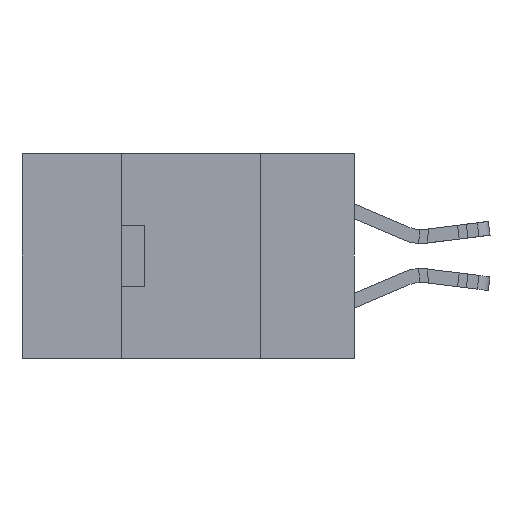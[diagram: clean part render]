
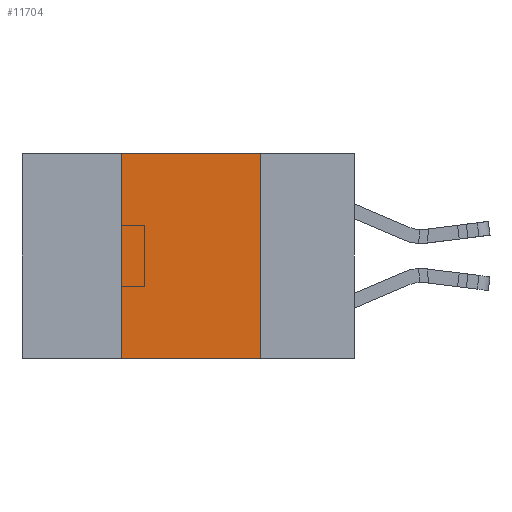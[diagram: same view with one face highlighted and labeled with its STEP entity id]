
A CAD part, left-side view. The second image highlights one B-rep face of the part: STEP entity #11704.
In plain terms, the highlighted planar face has unit normal (-1, 0, 0).
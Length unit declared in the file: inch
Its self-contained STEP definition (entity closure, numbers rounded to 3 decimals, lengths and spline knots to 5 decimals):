
#1423 = DIRECTION ( 'NONE',  ( 0., 0., -1. ) ) ;
#1690 = CARTESIAN_POINT ( 'NONE',  ( 0., 0.42, -0.37 ) ) ;
#1704 = DIRECTION ( 'NONE',  ( 1., 0., 0. ) ) ;
#2603 = EDGE_CURVE ( 'NONE', #26411, #3681, #3736, .T. ) ;
#2854 = VECTOR ( 'NONE', #8076, 39.37008 ) ;
#3369 = ORIENTED_EDGE ( 'NONE', *, *, #2603, .F. ) ;
#3681 = VERTEX_POINT ( 'NONE', #10088 ) ;
#3736 = LINE ( 'NONE', #18321, #10132 ) ;
#5758 = VERTEX_POINT ( 'NONE', #1690 ) ;
#5778 = FACE_OUTER_BOUND ( 'NONE', #7491, .T. ) ;
#6907 = LINE ( 'NONE', #15780, #23035 ) ;
#7236 = EDGE_CURVE ( 'NONE', #5758, #3681, #6907, .T. ) ;
#7491 = EDGE_LOOP ( 'NONE', ( #3369, #21550, #15401, #19804 ) ) ;
#8076 = DIRECTION ( 'NONE',  ( 0., -1., 0. ) ) ;
#8489 = CARTESIAN_POINT ( 'NONE',  ( 0., 0.42, -0.37 ) ) ;
#10088 = CARTESIAN_POINT ( 'NONE',  ( 0., 0.17, -0.37 ) ) ;
#10132 = VECTOR ( 'NONE', #19280, 39.37008 ) ;
#10551 = LINE ( 'NONE', #8489, #11176 ) ;
#11176 = VECTOR ( 'NONE', #13009, 39.37008 ) ;
#11704 = ADVANCED_FACE ( 'NONE', ( #5778 ), #12470, .F. ) ;
#12322 = CARTESIAN_POINT ( 'NONE',  ( 0., 0.17, 0. ) ) ;
#12470 = PLANE ( 'NONE',  #27787 ) ;
#12990 = VERTEX_POINT ( 'NONE', #17258 ) ;
#13009 = DIRECTION ( 'NONE',  ( 0., 0., 1. ) ) ;
#15401 = ORIENTED_EDGE ( 'NONE', *, *, #17916, .F. ) ;
#15780 = CARTESIAN_POINT ( 'NONE',  ( 0., 0.6, -0.37 ) ) ;
#17258 = CARTESIAN_POINT ( 'NONE',  ( 0., 0.42, 0. ) ) ;
#17916 = EDGE_CURVE ( 'NONE', #5758, #12990, #10551, .T. ) ;
#18321 = CARTESIAN_POINT ( 'NONE',  ( 0., 0.17, -0.37 ) ) ;
#19162 = EDGE_CURVE ( 'NONE', #12990, #26411, #28581, .T. ) ;
#19280 = DIRECTION ( 'NONE',  ( 0., 0., -1. ) ) ;
#19804 = ORIENTED_EDGE ( 'NONE', *, *, #7236, .T. ) ;
#21343 = CARTESIAN_POINT ( 'NONE',  ( 0., 0.6, 0. ) ) ;
#21550 = ORIENTED_EDGE ( 'NONE', *, *, #19162, .F. ) ;
#22469 = DIRECTION ( 'NONE',  ( 0., -1., 0. ) ) ;
#23035 = VECTOR ( 'NONE', #22469, 39.37008 ) ;
#24054 = CARTESIAN_POINT ( 'NONE',  ( 0., 0.6, 0. ) ) ;
#26411 = VERTEX_POINT ( 'NONE', #12322 ) ;
#27787 = AXIS2_PLACEMENT_3D ( 'NONE', #21343, #1704, #1423 ) ;
#28581 = LINE ( 'NONE', #24054, #2854 ) ;
